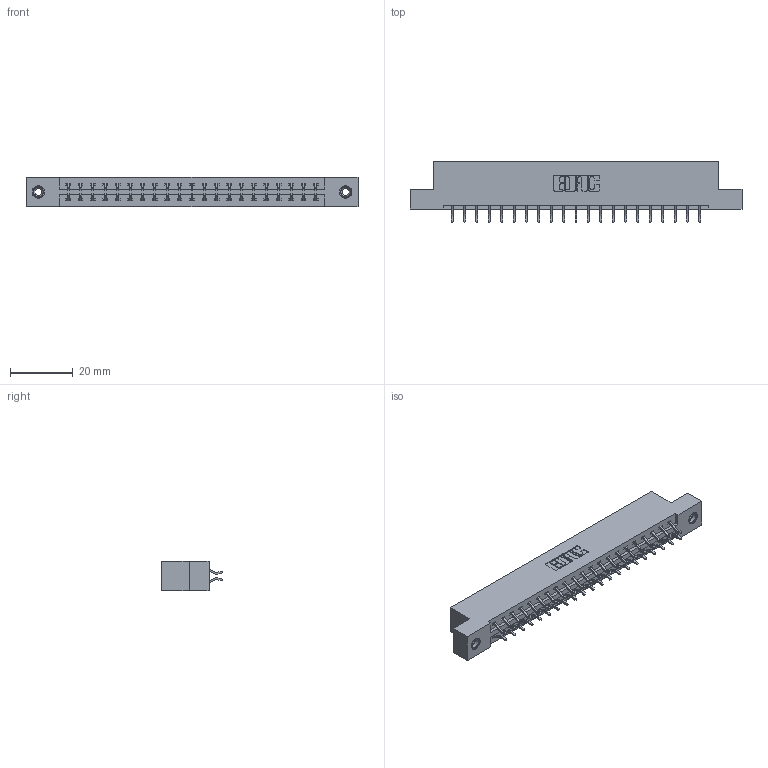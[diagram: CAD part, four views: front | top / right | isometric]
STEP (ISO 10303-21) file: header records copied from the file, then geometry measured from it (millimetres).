
FILE_DESCRIPTION (( 'STEP AP203' ), '1' );
FILE_NAME ('387-042-556-208.STEP', '2019-10-18T04:36:47', ( '' ), ( '' ), 'SwSTEP 2.0', 'SolidWorks 2016', '' );
FILE_SCHEMA (( 'CONFIG_CONTROL_DESIGN' ));
Length unit declared in the file: inch
Products named in the file (4): 345-292-001_556 Tail; 345-250-001_345-250-003-102; 337 Part_Flush Mounting Lugs - 0.156 Dia-TI; 387-042-556-208
Assembly tree (45 placements, depth 2):
  387-042-556-208
    337 Part_Flush Mounting Lugs - 0.156 Dia-TI
    345-292-001_556 Tail  x42
    345-250-001_345-250-003-102  x2
Bounding box: 106.22 x 19.57 x 9.4 mm (x, y, z)
Volume: 10906.9 mm3; surface area: 12105.9 mm2
Topology: 45 solids, 45 shells, 2694 faces, 7965 edges, 5246 vertices
Faces by surface type: plane 1866, cylinder 812, cone 12, torus 4
Entity records: 20404 total; most frequent: CARTESIAN_POINT 3449, ORIENTED_EDGE 3366, DIRECTION 2993, EDGE_CURVE 1683, LINE 1527, VECTOR 1527, VERTEX_POINT 1116, AXIS2_PLACEMENT_3D 733
